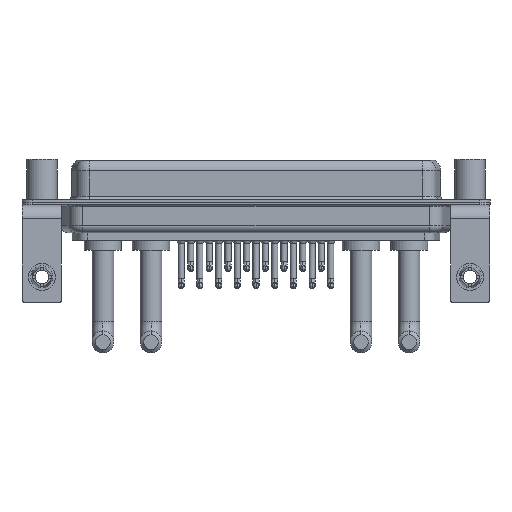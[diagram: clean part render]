
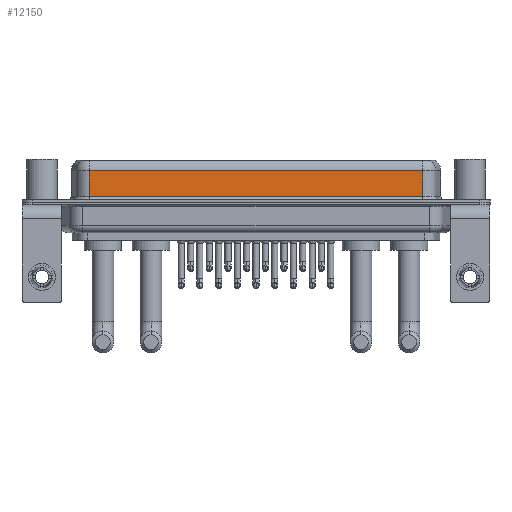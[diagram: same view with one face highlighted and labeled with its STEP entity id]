
A CAD part, front view. The second image highlights one B-rep face of the part: STEP entity #12150.
In plain terms, the highlighted planar face has unit normal (0, -1, 0).
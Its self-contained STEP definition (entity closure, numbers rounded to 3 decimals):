
#651 = FACE_OUTER_BOUND ( 'NONE', #21452, .T. ) ;
#1202 = DIRECTION ( 'NONE',  ( 0., 0., -1. ) ) ;
#2584 = DIRECTION ( 'NONE',  ( 0., 0., 1. ) ) ;
#3372 = VECTOR ( 'NONE', #19203, 1000. ) ;
#4286 = LINE ( 'NONE', #22469, #22185 ) ;
#4418 = DIRECTION ( 'NONE',  ( -1., 0., 0. ) ) ;
#5110 = CARTESIAN_POINT ( 'NONE',  ( 7.038, -3.95, 6.4 ) ) ;
#5374 = LINE ( 'NONE', #17485, #7601 ) ;
#5512 = DIRECTION ( 'NONE',  ( 0., 0., -1. ) ) ;
#6090 = ORIENTED_EDGE ( 'NONE', *, *, #20676, .T. ) ;
#6155 = ORIENTED_EDGE ( 'NONE', *, *, #15484, .F. ) ;
#6448 = VERTEX_POINT ( 'NONE', #12057 ) ;
#7601 = VECTOR ( 'NONE', #5512, 1000. ) ;
#8362 = VECTOR ( 'NONE', #1202, 1000. ) ;
#9269 = EDGE_CURVE ( 'NONE', #19554, #24175, #9906, .T. ) ;
#9586 = EDGE_CURVE ( 'NONE', #17309, #19554, #22786, .T. ) ;
#9769 = PLANE ( 'NONE',  #12571 ) ;
#9906 = LINE ( 'NONE', #23590, #3372 ) ;
#12057 = CARTESIAN_POINT ( 'NONE',  ( 56.462, -3.95, 4.65 ) ) ;
#12150 = ADVANCED_FACE ( 'NONE', ( #651 ), #9769, .F. ) ;
#12381 = ORIENTED_EDGE ( 'NONE', *, *, #9269, .T. ) ;
#12571 = AXIS2_PLACEMENT_3D ( 'NONE', #25516, #19441, #2584 ) ;
#13172 = ORIENTED_EDGE ( 'NONE', *, *, #9586, .T. ) ;
#15484 = EDGE_CURVE ( 'NONE', #6448, #24175, #5374, .T. ) ;
#17309 = VERTEX_POINT ( 'NONE', #20382 ) ;
#17485 = CARTESIAN_POINT ( 'NONE',  ( 56.462, -3.95, 6.4 ) ) ;
#17886 = CARTESIAN_POINT ( 'NONE',  ( 7.038, -3.95, 0.9 ) ) ;
#19203 = DIRECTION ( 'NONE',  ( 1., 0., 0. ) ) ;
#19441 = DIRECTION ( 'NONE',  ( 0., 1., 0. ) ) ;
#19554 = VERTEX_POINT ( 'NONE', #17886 ) ;
#20382 = CARTESIAN_POINT ( 'NONE',  ( 7.038, -3.95, 4.65 ) ) ;
#20676 = EDGE_CURVE ( 'NONE', #6448, #17309, #4286, .T. ) ;
#21452 = EDGE_LOOP ( 'NONE', ( #6155, #6090, #13172, #12381 ) ) ;
#21462 = CARTESIAN_POINT ( 'NONE',  ( 56.462, -3.95, 0.9 ) ) ;
#22185 = VECTOR ( 'NONE', #4418, 1000. ) ;
#22469 = CARTESIAN_POINT ( 'NONE',  ( 56.462, -3.95, 4.65 ) ) ;
#22786 = LINE ( 'NONE', #5110, #8362 ) ;
#23590 = CARTESIAN_POINT ( 'NONE',  ( 56.462, -3.95, 0.9 ) ) ;
#24175 = VERTEX_POINT ( 'NONE', #21462 ) ;
#25516 = CARTESIAN_POINT ( 'NONE',  ( 56.462, -3.95, 6.4 ) ) ;
